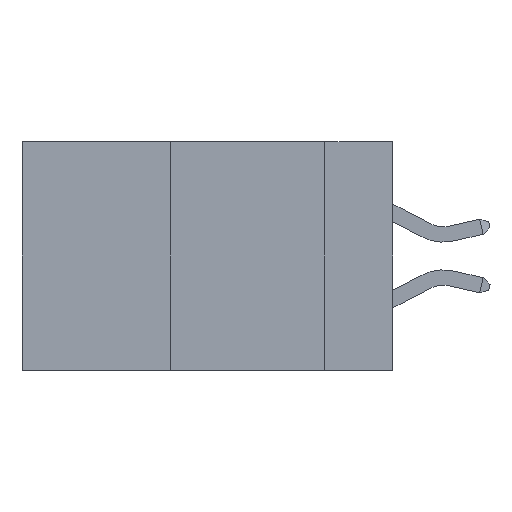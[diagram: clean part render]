
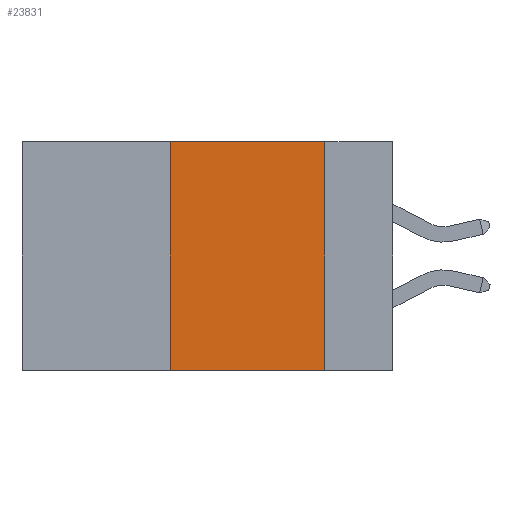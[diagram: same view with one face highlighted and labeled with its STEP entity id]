
A CAD part, left-side view. The second image highlights one B-rep face of the part: STEP entity #23831.
In plain terms, the highlighted planar face has unit normal (-1, 0, 0).
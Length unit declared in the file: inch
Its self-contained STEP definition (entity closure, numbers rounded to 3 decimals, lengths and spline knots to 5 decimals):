
#224 = DIRECTION ( 'NONE',  ( 0., 0., -1. ) ) ;
#427 = CARTESIAN_POINT ( 'NONE',  ( 0., 0.36, -0.37 ) ) ;
#2813 = FACE_OUTER_BOUND ( 'NONE', #4172, .T. ) ;
#3032 = ORIENTED_EDGE ( 'NONE', *, *, #5538, .T. ) ;
#3043 = VECTOR ( 'NONE', #6157, 39.37008 ) ;
#3086 = CARTESIAN_POINT ( 'NONE',  ( 0., 0.6, 0. ) ) ;
#3537 = CARTESIAN_POINT ( 'NONE',  ( 0., 0.36, 0. ) ) ;
#4172 = EDGE_LOOP ( 'NONE', ( #15089, #4553, #20719, #3032 ) ) ;
#4553 = ORIENTED_EDGE ( 'NONE', *, *, #14945, .F. ) ;
#5538 = EDGE_CURVE ( 'NONE', #18582, #12527, #18689, .T. ) ;
#6092 = CARTESIAN_POINT ( 'NONE',  ( 0., 0.11, -0.37 ) ) ;
#6157 = DIRECTION ( 'NONE',  ( 0., -1., 0. ) ) ;
#7540 = PLANE ( 'NONE',  #22432 ) ;
#8409 = CARTESIAN_POINT ( 'NONE',  ( 0., 0.11, 0. ) ) ;
#8605 = VECTOR ( 'NONE', #17618, 39.37008 ) ;
#9821 = DIRECTION ( 'NONE',  ( 1., 0., 0. ) ) ;
#10723 = LINE ( 'NONE', #8409, #8605 ) ;
#11404 = CARTESIAN_POINT ( 'NONE',  ( 0., 0.36, 0. ) ) ;
#11470 = EDGE_CURVE ( 'NONE', #18582, #11512, #24953, .T. ) ;
#11512 = VERTEX_POINT ( 'NONE', #11404 ) ;
#12092 = CARTESIAN_POINT ( 'NONE',  ( 0., 0.6, 0. ) ) ;
#12527 = VERTEX_POINT ( 'NONE', #6092 ) ;
#14307 = DIRECTION ( 'NONE',  ( 0., -1., 0. ) ) ;
#14945 = EDGE_CURVE ( 'NONE', #11512, #27783, #17307, .T. ) ;
#15089 = ORIENTED_EDGE ( 'NONE', *, *, #29382, .F. ) ;
#16797 = VECTOR ( 'NONE', #19515, 39.37008 ) ;
#17307 = LINE ( 'NONE', #3086, #21547 ) ;
#17618 = DIRECTION ( 'NONE',  ( 0., 0., -1. ) ) ;
#17655 = CARTESIAN_POINT ( 'NONE',  ( 0., 0.6, -0.37 ) ) ;
#18582 = VERTEX_POINT ( 'NONE', #427 ) ;
#18689 = LINE ( 'NONE', #17655, #3043 ) ;
#19515 = DIRECTION ( 'NONE',  ( 0., 0., 1. ) ) ;
#20719 = ORIENTED_EDGE ( 'NONE', *, *, #11470, .F. ) ;
#21547 = VECTOR ( 'NONE', #14307, 39.37008 ) ;
#22432 = AXIS2_PLACEMENT_3D ( 'NONE', #12092, #9821, #224 ) ;
#23831 = ADVANCED_FACE ( 'NONE', ( #2813 ), #7540, .F. ) ;
#24953 = LINE ( 'NONE', #3537, #16797 ) ;
#27483 = CARTESIAN_POINT ( 'NONE',  ( 0., 0.11, 0. ) ) ;
#27783 = VERTEX_POINT ( 'NONE', #27483 ) ;
#29382 = EDGE_CURVE ( 'NONE', #27783, #12527, #10723, .T. ) ;
